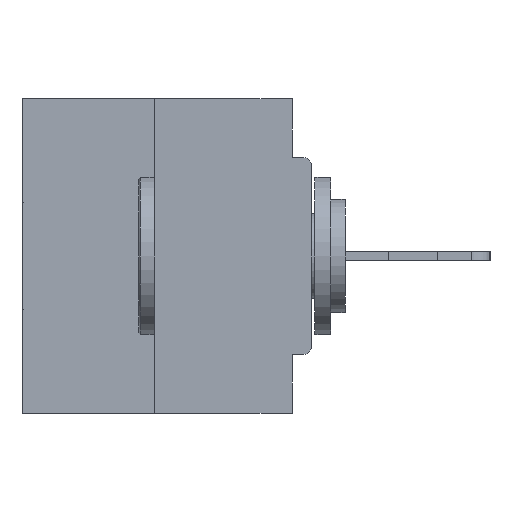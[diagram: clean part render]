
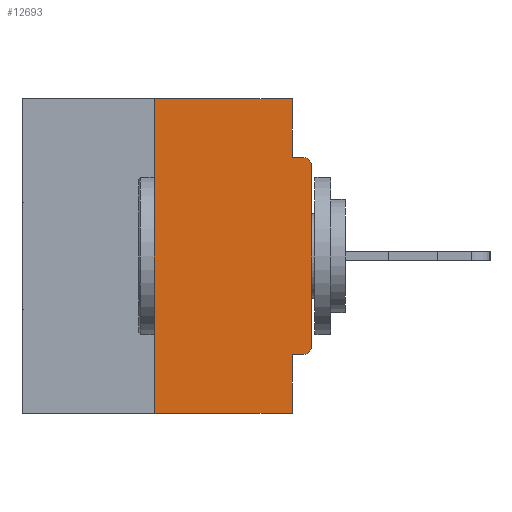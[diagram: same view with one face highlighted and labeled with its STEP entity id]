
A CAD part, left-side view. The second image highlights one B-rep face of the part: STEP entity #12693.
In plain terms, the highlighted planar face has unit normal (-1, 0, 0).
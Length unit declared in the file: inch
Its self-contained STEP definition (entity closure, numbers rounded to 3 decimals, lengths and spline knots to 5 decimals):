
#437 = VERTEX_POINT ( 'NONE', #24274 ) ;
#1309 = DIRECTION ( 'NONE',  ( 0., 0., 1. ) ) ;
#1384 = VERTEX_POINT ( 'NONE', #25502 ) ;
#1738 = VERTEX_POINT ( 'NONE', #25679 ) ;
#2371 = VERTEX_POINT ( 'NONE', #17659 ) ;
#2534 = LINE ( 'NONE', #30890, #16416 ) ;
#3172 = CARTESIAN_POINT ( 'NONE',  ( 0., 0., 0. ) ) ;
#3564 = EDGE_CURVE ( 'NONE', #5446, #2371, #29220, .T. ) ;
#3797 = DIRECTION ( 'NONE',  ( -1., 0., 0. ) ) ;
#4250 = ORIENTED_EDGE ( 'NONE', *, *, #15158, .T. ) ;
#4823 = EDGE_CURVE ( 'NONE', #29609, #14805, #11756, .T. ) ;
#4968 = PLANE ( 'NONE',  #8909 ) ;
#5446 = VERTEX_POINT ( 'NONE', #23515 ) ;
#5545 = VERTEX_POINT ( 'NONE', #19432 ) ;
#6049 = AXIS2_PLACEMENT_3D ( 'NONE', #20413, #3797, #23153 ) ;
#6489 = ORIENTED_EDGE ( 'NONE', *, *, #3564, .T. ) ;
#7181 = VECTOR ( 'NONE', #15375, 39.37008 ) ;
#7754 = DIRECTION ( 'NONE',  ( 0., 0., -1. ) ) ;
#7795 = EDGE_CURVE ( 'NONE', #30108, #10763, #35018, .T. ) ;
#8774 = CIRCLE ( 'NONE', #6049, 0.015 ) ;
#8909 = AXIS2_PLACEMENT_3D ( 'NONE', #13197, #24312, #7754 ) ;
#9559 = DIRECTION ( 'NONE',  ( -1., 0., 0. ) ) ;
#10763 = VERTEX_POINT ( 'NONE', #26116 ) ;
#10881 = VECTOR ( 'NONE', #15152, 39.37008 ) ;
#11756 = LINE ( 'NONE', #13554, #32755 ) ;
#12037 = VECTOR ( 'NONE', #23345, 39.37008 ) ;
#12693 = ADVANCED_FACE ( 'NONE', ( #34610 ), #4968, .F. ) ;
#13197 = CARTESIAN_POINT ( 'NONE',  ( 0., 0.46, 0. ) ) ;
#13358 = DIRECTION ( 'NONE',  ( 0., -1., 0. ) ) ;
#13554 = CARTESIAN_POINT ( 'NONE',  ( 0., 0.46, 0. ) ) ;
#14453 = ORIENTED_EDGE ( 'NONE', *, *, #34123, .F. ) ;
#14606 = VECTOR ( 'NONE', #1309, 39.37008 ) ;
#14805 = VERTEX_POINT ( 'NONE', #32613 ) ;
#15152 = DIRECTION ( 'NONE',  ( 0., 1., 0. ) ) ;
#15158 = EDGE_CURVE ( 'NONE', #437, #5446, #31521, .T. ) ;
#15257 = CARTESIAN_POINT ( 'NONE',  ( 0., 0.25, 0. ) ) ;
#15375 = DIRECTION ( 'NONE',  ( 0., 0., 1. ) ) ;
#16342 = CARTESIAN_POINT ( 'NONE',  ( 0., 0., -0.0935 ) ) ;
#16416 = VECTOR ( 'NONE', #33562, 39.37008 ) ;
#16977 = CARTESIAN_POINT ( 'NONE',  ( 0., 0.25, -0.5 ) ) ;
#17659 = CARTESIAN_POINT ( 'NONE',  ( 0., 0., -0.1085 ) ) ;
#18228 = LINE ( 'NONE', #28745, #10881 ) ;
#18271 = AXIS2_PLACEMENT_3D ( 'NONE', #26108, #9559, #28848 ) ;
#18302 = CARTESIAN_POINT ( 'NONE',  ( 0., 0.46, -0.5 ) ) ;
#18852 = DIRECTION ( 'NONE',  ( 0., -1., 0. ) ) ;
#18991 = EDGE_CURVE ( 'NONE', #2371, #1384, #8774, .T. ) ;
#19432 = CARTESIAN_POINT ( 'NONE',  ( 0., 0.031, -0.0935 ) ) ;
#19443 = LINE ( 'NONE', #20599, #12037 ) ;
#20029 = CARTESIAN_POINT ( 'NONE',  ( 0., 0.25, 0. ) ) ;
#20413 = CARTESIAN_POINT ( 'NONE',  ( 0., 0.015, -0.1085 ) ) ;
#20599 = CARTESIAN_POINT ( 'NONE',  ( 0., 0.031, 0. ) ) ;
#20641 = VECTOR ( 'NONE', #18852, 39.37008 ) ;
#21339 = EDGE_CURVE ( 'NONE', #1738, #10763, #2534, .T. ) ;
#21568 = LINE ( 'NONE', #16342, #27153 ) ;
#22794 = LINE ( 'NONE', #15257, #7181 ) ;
#23153 = DIRECTION ( 'NONE',  ( 0., 0., -1. ) ) ;
#23326 = EDGE_CURVE ( 'NONE', #437, #1738, #18228, .T. ) ;
#23345 = DIRECTION ( 'NONE',  ( 0., 0., -1. ) ) ;
#23515 = CARTESIAN_POINT ( 'NONE',  ( 0., 0., -0.3915 ) ) ;
#24274 = CARTESIAN_POINT ( 'NONE',  ( 0., 0.015, -0.4065 ) ) ;
#24312 = DIRECTION ( 'NONE',  ( 1., 0., 0. ) ) ;
#24678 = DIRECTION ( 'NONE',  ( 0., -1., 0. ) ) ;
#24740 = ORIENTED_EDGE ( 'NONE', *, *, #18991, .T. ) ;
#25479 = ORIENTED_EDGE ( 'NONE', *, *, #23326, .F. ) ;
#25502 = CARTESIAN_POINT ( 'NONE',  ( 0., 0.015, -0.0935 ) ) ;
#25580 = EDGE_CURVE ( 'NONE', #5545, #1384, #21568, .T. ) ;
#25679 = CARTESIAN_POINT ( 'NONE',  ( 0., 0.031, -0.4065 ) ) ;
#26108 = CARTESIAN_POINT ( 'NONE',  ( 0., 0.015, -0.3915 ) ) ;
#26116 = CARTESIAN_POINT ( 'NONE',  ( 0., 0.031, -0.5 ) ) ;
#26243 = ORIENTED_EDGE ( 'NONE', *, *, #25580, .F. ) ;
#27153 = VECTOR ( 'NONE', #24678, 39.37008 ) ;
#27272 = ORIENTED_EDGE ( 'NONE', *, *, #21339, .F. ) ;
#27293 = ORIENTED_EDGE ( 'NONE', *, *, #7795, .T. ) ;
#28745 = CARTESIAN_POINT ( 'NONE',  ( 0., 0., -0.4065 ) ) ;
#28848 = DIRECTION ( 'NONE',  ( 0., 0., -1. ) ) ;
#29220 = LINE ( 'NONE', #3172, #14606 ) ;
#29609 = VERTEX_POINT ( 'NONE', #20029 ) ;
#30108 = VERTEX_POINT ( 'NONE', #16977 ) ;
#30890 = CARTESIAN_POINT ( 'NONE',  ( 0., 0.031, -0.5 ) ) ;
#30967 = ORIENTED_EDGE ( 'NONE', *, *, #32307, .F. ) ;
#31521 = CIRCLE ( 'NONE', #18271, 0.015 ) ;
#32307 = EDGE_CURVE ( 'NONE', #14805, #5545, #19443, .T. ) ;
#32429 = ORIENTED_EDGE ( 'NONE', *, *, #4823, .F. ) ;
#32613 = CARTESIAN_POINT ( 'NONE',  ( 0., 0.031, 0. ) ) ;
#32628 = EDGE_LOOP ( 'NONE', ( #32429, #14453, #27293, #27272, #25479, #4250, #6489, #24740, #26243, #30967 ) ) ;
#32755 = VECTOR ( 'NONE', #13358, 39.37008 ) ;
#33562 = DIRECTION ( 'NONE',  ( 0., 0., -1. ) ) ;
#34123 = EDGE_CURVE ( 'NONE', #30108, #29609, #22794, .T. ) ;
#34610 = FACE_OUTER_BOUND ( 'NONE', #32628, .T. ) ;
#35018 = LINE ( 'NONE', #18302, #20641 ) ;
